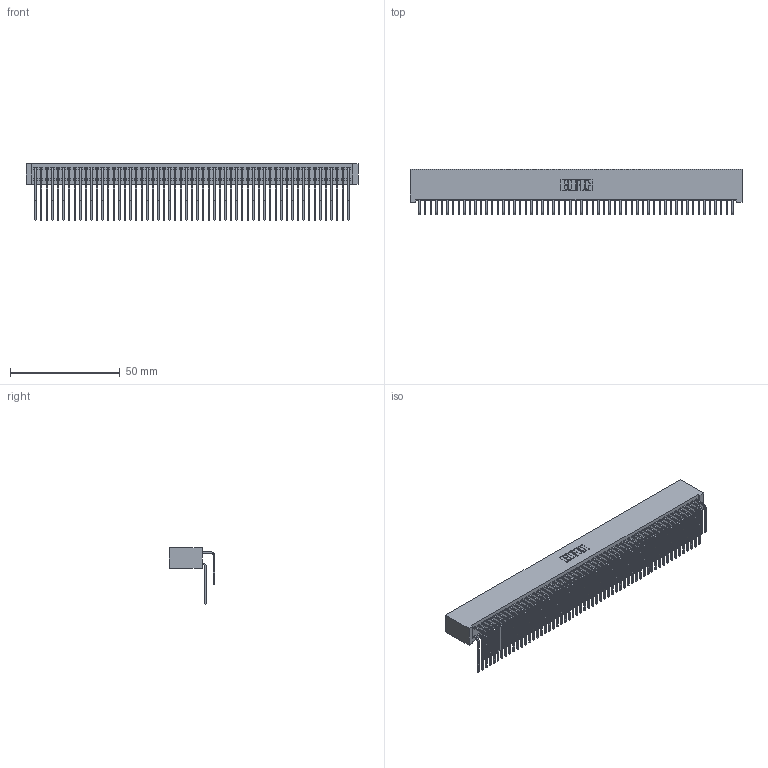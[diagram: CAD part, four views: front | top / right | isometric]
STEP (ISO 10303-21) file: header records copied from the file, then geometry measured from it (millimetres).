
FILE_DESCRIPTION (( 'STEP AP203' ), '1' );
FILE_NAME ('342-114-559-201.STEP', '2019-10-04T21:50:49', ( '' ), ( '' ), 'SwSTEP 2.0', 'SolidWorks 2016', '' );
FILE_SCHEMA (( 'CONFIG_CONTROL_DESIGN' ));
Length unit declared in the file: inch
Products named in the file (4): 342 Part_Lugless; 345-292-001_558 559 Tail - 1; 345-292-001_559 Tail - 2; 342-114-559-201
Assembly tree (115 placements, depth 2):
  342-114-559-201
    342 Part_Lugless
    345-292-001_558 559 Tail - 1  x57
    345-292-001_559 Tail - 2  x57
Bounding box: 151.03 x 20.64 x 25.78 mm (x, y, z)
Volume: 14738 mm3; surface area: 27780.6 mm2
Topology: 115 solids, 115 shells, 6258 faces, 18629 edges, 12266 vertices
Faces by surface type: plane 4394, cylinder 1864
Entity records: 36105 total; most frequent: CARTESIAN_POINT 6013, ORIENTED_EDGE 5898, DIRECTION 5085, EDGE_CURVE 2949, LINE 2789, VECTOR 2789, VERTEX_POINT 1962, AXIS2_PLACEMENT_3D 1148
